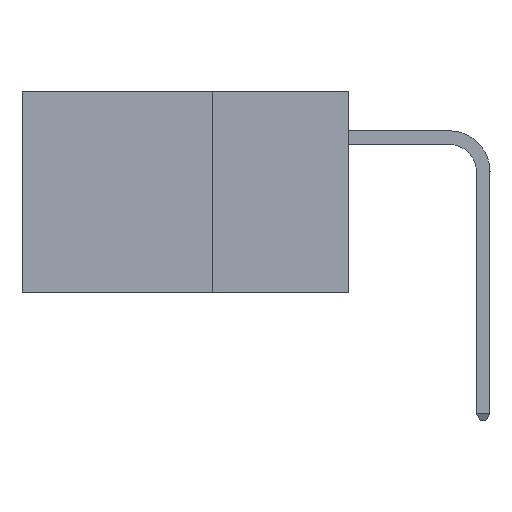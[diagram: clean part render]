
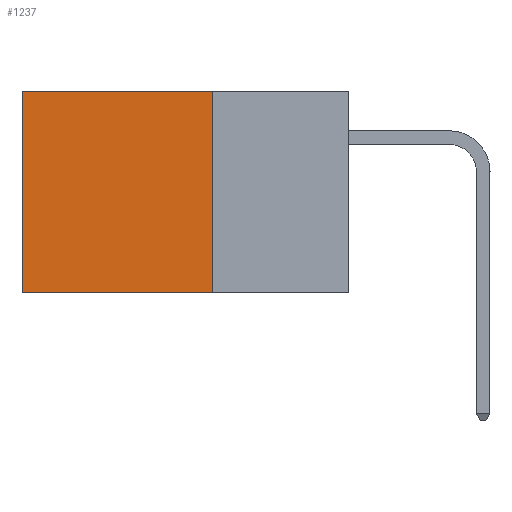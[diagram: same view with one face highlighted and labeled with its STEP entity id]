
A CAD part, left-side view. The second image highlights one B-rep face of the part: STEP entity #1237.
In plain terms, the highlighted planar face has unit normal (-1, 0, 0).
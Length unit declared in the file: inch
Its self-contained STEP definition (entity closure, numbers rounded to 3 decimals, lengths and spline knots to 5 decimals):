
#727 = DIRECTION ( 'NONE',  ( 0., 0., -1. ) ) ;
#825 = DIRECTION ( 'NONE',  ( 1., 0., 0. ) ) ;
#1040 = EDGE_CURVE ( 'NONE', #10782, #6497, #12961, .T. ) ;
#1237 = ADVANCED_FACE ( 'NONE', ( #16534 ), #2216, .F. ) ;
#1295 = CARTESIAN_POINT ( 'NONE',  ( 0.2875, 0.25, 0. ) ) ;
#2054 = VECTOR ( 'NONE', #9716, 39.37008 ) ;
#2182 = EDGE_CURVE ( 'NONE', #7392, #6497, #2739, .T. ) ;
#2216 = PLANE ( 'NONE',  #7864 ) ;
#2739 = LINE ( 'NONE', #13116, #16502 ) ;
#2741 = ORIENTED_EDGE ( 'NONE', *, *, #1040, .F. ) ;
#2824 = CARTESIAN_POINT ( 'NONE',  ( 0.2875, 0.25, 0. ) ) ;
#3946 = DIRECTION ( 'NONE',  ( 0., 0., -1. ) ) ;
#4306 = DIRECTION ( 'NONE',  ( 0., 1., 0. ) ) ;
#4643 = EDGE_LOOP ( 'NONE', ( #7300, #2741, #16034, #8887 ) ) ;
#5353 = DIRECTION ( 'NONE',  ( 0., 1., 0. ) ) ;
#5771 = LINE ( 'NONE', #1295, #2054 ) ;
#6497 = VERTEX_POINT ( 'NONE', #8098 ) ;
#7043 = CARTESIAN_POINT ( 'NONE',  ( 0.2875, 0.25, -0.37 ) ) ;
#7300 = ORIENTED_EDGE ( 'NONE', *, *, #2182, .T. ) ;
#7392 = VERTEX_POINT ( 'NONE', #7637 ) ;
#7637 = CARTESIAN_POINT ( 'NONE',  ( 0.2875, 0.6, 0. ) ) ;
#7757 = EDGE_CURVE ( 'NONE', #13979, #10782, #5771, .T. ) ;
#7864 = AXIS2_PLACEMENT_3D ( 'NONE', #2824, #825, #727 ) ;
#8098 = CARTESIAN_POINT ( 'NONE',  ( 0.2875, 0.6, -0.37 ) ) ;
#8375 = CARTESIAN_POINT ( 'NONE',  ( 0.2875, 0.25, 0. ) ) ;
#8887 = ORIENTED_EDGE ( 'NONE', *, *, #11613, .T. ) ;
#9716 = DIRECTION ( 'NONE',  ( 0., 0., -1. ) ) ;
#10782 = VERTEX_POINT ( 'NONE', #15770 ) ;
#11116 = CARTESIAN_POINT ( 'NONE',  ( 0.2875, 0.25, 0. ) ) ;
#11613 = EDGE_CURVE ( 'NONE', #13979, #7392, #13010, .T. ) ;
#12543 = VECTOR ( 'NONE', #5353, 39.37008 ) ;
#12961 = LINE ( 'NONE', #7043, #12543 ) ;
#13010 = LINE ( 'NONE', #11116, #15582 ) ;
#13116 = CARTESIAN_POINT ( 'NONE',  ( 0.2875, 0.6, 0. ) ) ;
#13979 = VERTEX_POINT ( 'NONE', #8375 ) ;
#15582 = VECTOR ( 'NONE', #4306, 39.37008 ) ;
#15770 = CARTESIAN_POINT ( 'NONE',  ( 0.2875, 0.25, -0.37 ) ) ;
#16034 = ORIENTED_EDGE ( 'NONE', *, *, #7757, .F. ) ;
#16502 = VECTOR ( 'NONE', #3946, 39.37008 ) ;
#16534 = FACE_OUTER_BOUND ( 'NONE', #4643, .T. ) ;
